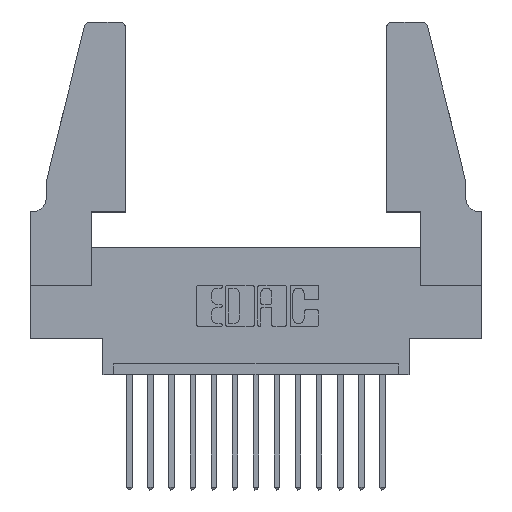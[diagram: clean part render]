
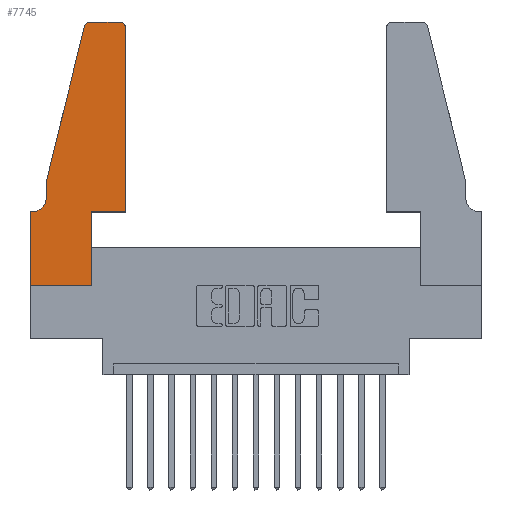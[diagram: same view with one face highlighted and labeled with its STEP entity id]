
A CAD part, top view. The second image highlights one B-rep face of the part: STEP entity #7745.
In plain terms, the highlighted planar face has unit normal (0, 0, 1).
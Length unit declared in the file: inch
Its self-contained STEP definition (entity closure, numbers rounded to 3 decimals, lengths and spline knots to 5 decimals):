
#63 = LINE ( 'NONE', #11155, #7960 ) ;
#189 = DIRECTION ( 'NONE',  ( 1., 0., 0. ) ) ;
#231 = ORIENTED_EDGE ( 'NONE', *, *, #7667, .T. ) ;
#413 = EDGE_CURVE ( 'NONE', #4228, #542, #7952, .T. ) ;
#529 = DIRECTION ( 'NONE',  ( -1., 0., 0. ) ) ;
#542 = VERTEX_POINT ( 'NONE', #15100 ) ;
#608 = EDGE_CURVE ( 'NONE', #13266, #11403, #9667, .T. ) ;
#725 = LINE ( 'NONE', #15301, #3039 ) ;
#782 = VECTOR ( 'NONE', #9727, 39.37008 ) ;
#928 = DIRECTION ( 'NONE',  ( 0., 0., 1. ) ) ;
#932 = AXIS2_PLACEMENT_3D ( 'NONE', #10779, #1033, #7289 ) ;
#1033 = DIRECTION ( 'NONE',  ( 0., 0., 1. ) ) ;
#1196 = DIRECTION ( 'NONE',  ( 0., -1., 0. ) ) ;
#1486 = VERTEX_POINT ( 'NONE', #13986 ) ;
#1506 = ORIENTED_EDGE ( 'NONE', *, *, #13818, .T. ) ;
#1510 = VECTOR ( 'NONE', #1196, 39.37008 ) ;
#1720 = DIRECTION ( 'NONE',  ( 0., 1., 0. ) ) ;
#1723 = VECTOR ( 'NONE', #12446, 39.37008 ) ;
#1784 = DIRECTION ( 'NONE',  ( 0., 0., -1. ) ) ;
#2279 = DIRECTION ( 'NONE',  ( 0., 1., 0. ) ) ;
#2294 = LINE ( 'NONE', #2817, #1723 ) ;
#2319 = CARTESIAN_POINT ( 'NONE',  ( 0.284, 1.22, 0.37 ) ) ;
#2699 = PLANE ( 'NONE',  #932 ) ;
#2817 = CARTESIAN_POINT ( 'NONE',  ( 0., 0., 0.37 ) ) ;
#2874 = LINE ( 'NONE', #2894, #12319 ) ;
#2894 = CARTESIAN_POINT ( 'NONE',  ( 0.4505, 0.35, 0.37 ) ) ;
#3039 = VECTOR ( 'NONE', #529, 39.37008 ) ;
#3141 = CARTESIAN_POINT ( 'NONE',  ( 0.2865, 0., 0.37 ) ) ;
#3272 = LINE ( 'NONE', #9671, #782 ) ;
#3279 = VERTEX_POINT ( 'NONE', #13109 ) ;
#3330 = CARTESIAN_POINT ( 'NONE',  ( 0.2865, 0.35, 0.37 ) ) ;
#3629 = CIRCLE ( 'NONE', #12653, 0.03 ) ;
#3825 = ORIENTED_EDGE ( 'NONE', *, *, #15422, .T. ) ;
#4015 = CARTESIAN_POINT ( 'NONE',  ( 0.0755, 0.5, 0.37 ) ) ;
#4043 = DIRECTION ( 'NONE',  ( -1., 0., 0. ) ) ;
#4045 = VERTEX_POINT ( 'NONE', #4311 ) ;
#4228 = VERTEX_POINT ( 'NONE', #7451 ) ;
#4311 = CARTESIAN_POINT ( 'NONE',  ( 0.4205, 1.25, 0.37 ) ) ;
#4902 = ORIENTED_EDGE ( 'NONE', *, *, #12905, .T. ) ;
#4983 = AXIS2_PLACEMENT_3D ( 'NONE', #2319, #928, #12179 ) ;
#5241 = EDGE_CURVE ( 'NONE', #542, #13461, #63, .T. ) ;
#5248 = CARTESIAN_POINT ( 'NONE',  ( 0.4205, 1.22, 0.37 ) ) ;
#5386 = LINE ( 'NONE', #8455, #1510 ) ;
#5908 = LINE ( 'NONE', #15460, #12884 ) ;
#6015 = DIRECTION ( 'NONE',  ( -0.239, -0.971, 0. ) ) ;
#6518 = FACE_OUTER_BOUND ( 'NONE', #14135, .T. ) ;
#7149 = CARTESIAN_POINT ( 'NONE',  ( 0.4505, 0.35, 0.37 ) ) ;
#7289 = DIRECTION ( 'NONE',  ( 1., 0., 0. ) ) ;
#7338 = ORIENTED_EDGE ( 'NONE', *, *, #13705, .T. ) ;
#7344 = ORIENTED_EDGE ( 'NONE', *, *, #12371, .T. ) ;
#7451 = CARTESIAN_POINT ( 'NONE',  ( 0.284, 1.25, 0.37 ) ) ;
#7667 = EDGE_CURVE ( 'NONE', #12874, #9202, #3272, .T. ) ;
#7682 = AXIS2_PLACEMENT_3D ( 'NONE', #9146, #1784, #15384 ) ;
#7745 = ADVANCED_FACE ( 'NONE', ( #6518 ), #2699, .T. ) ;
#7828 = DIRECTION ( 'NONE',  ( 1., 0., 0. ) ) ;
#7952 = CIRCLE ( 'NONE', #4983, 0.03 ) ;
#7960 = VECTOR ( 'NONE', #6015, 39.37008 ) ;
#8149 = VECTOR ( 'NONE', #1720, 39.37008 ) ;
#8455 = CARTESIAN_POINT ( 'NONE',  ( 0.0755, 0.5, 0.37 ) ) ;
#8996 = VERTEX_POINT ( 'NONE', #15156 ) ;
#9056 = ORIENTED_EDGE ( 'NONE', *, *, #12890, .T. ) ;
#9146 = CARTESIAN_POINT ( 'NONE',  ( 0.0055, 0.42, 0.37 ) ) ;
#9202 = VERTEX_POINT ( 'NONE', #11479 ) ;
#9304 = CARTESIAN_POINT ( 'NONE',  ( 0.4505, 1.22, 0.37 ) ) ;
#9667 = LINE ( 'NONE', #3330, #8149 ) ;
#9671 = CARTESIAN_POINT ( 'NONE',  ( 0., 0., 0.37 ) ) ;
#9727 = DIRECTION ( 'NONE',  ( 0., -1., 0. ) ) ;
#10391 = VECTOR ( 'NONE', #2279, 39.37008 ) ;
#10779 = CARTESIAN_POINT ( 'NONE',  ( 0., 0.35, 0.37 ) ) ;
#11059 = ORIENTED_EDGE ( 'NONE', *, *, #608, .T. ) ;
#11155 = CARTESIAN_POINT ( 'NONE',  ( 0.0755, 0.5, 0.37 ) ) ;
#11343 = CARTESIAN_POINT ( 'NONE',  ( 0., 0.35, 0.37 ) ) ;
#11390 = ORIENTED_EDGE ( 'NONE', *, *, #5241, .T. ) ;
#11403 = VERTEX_POINT ( 'NONE', #13115 ) ;
#11468 = VERTEX_POINT ( 'NONE', #9304 ) ;
#11479 = CARTESIAN_POINT ( 'NONE',  ( 0., 0., 0.37 ) ) ;
#11537 = ORIENTED_EDGE ( 'NONE', *, *, #12830, .T. ) ;
#12179 = DIRECTION ( 'NONE',  ( 1., 0., 0. ) ) ;
#12319 = VECTOR ( 'NONE', #7828, 39.37008 ) ;
#12371 = EDGE_CURVE ( 'NONE', #3279, #1486, #14083, .T. ) ;
#12422 = DIRECTION ( 'NONE',  ( 0., 0., 1. ) ) ;
#12446 = DIRECTION ( 'NONE',  ( 1., 0., 0. ) ) ;
#12506 = LINE ( 'NONE', #7149, #10391 ) ;
#12653 = AXIS2_PLACEMENT_3D ( 'NONE', #5248, #12422, #189 ) ;
#12830 = EDGE_CURVE ( 'NONE', #13461, #3279, #5386, .T. ) ;
#12874 = VERTEX_POINT ( 'NONE', #11343 ) ;
#12884 = VECTOR ( 'NONE', #4043, 39.37008 ) ;
#12890 = EDGE_CURVE ( 'NONE', #9202, #13266, #2294, .T. ) ;
#12905 = EDGE_CURVE ( 'NONE', #8996, #11468, #12506, .T. ) ;
#13109 = CARTESIAN_POINT ( 'NONE',  ( 0.0755, 0.42, 0.37 ) ) ;
#13115 = CARTESIAN_POINT ( 'NONE',  ( 0.2865, 0.35, 0.37 ) ) ;
#13266 = VERTEX_POINT ( 'NONE', #3141 ) ;
#13461 = VERTEX_POINT ( 'NONE', #4015 ) ;
#13609 = EDGE_CURVE ( 'NONE', #11468, #4045, #3629, .T. ) ;
#13705 = EDGE_CURVE ( 'NONE', #4045, #4228, #5908, .T. ) ;
#13818 = EDGE_CURVE ( 'NONE', #1486, #12874, #725, .T. ) ;
#13986 = CARTESIAN_POINT ( 'NONE',  ( 0.0055, 0.35, 0.37 ) ) ;
#14083 = CIRCLE ( 'NONE', #7682, 0.07 ) ;
#14135 = EDGE_LOOP ( 'NONE', ( #7338, #15339, #11390, #11537, #7344, #1506, #231, #9056, #11059, #3825, #4902, #14521 ) ) ;
#14521 = ORIENTED_EDGE ( 'NONE', *, *, #13609, .T. ) ;
#15100 = CARTESIAN_POINT ( 'NONE',  ( 0.25487, 1.22718, 0.37 ) ) ;
#15156 = CARTESIAN_POINT ( 'NONE',  ( 0.4505, 0.35, 0.37 ) ) ;
#15301 = CARTESIAN_POINT ( 'NONE',  ( 0.0755, 0.35, 0.37 ) ) ;
#15339 = ORIENTED_EDGE ( 'NONE', *, *, #413, .T. ) ;
#15384 = DIRECTION ( 'NONE',  ( -1., 0., 0. ) ) ;
#15422 = EDGE_CURVE ( 'NONE', #11403, #8996, #2874, .T. ) ;
#15460 = CARTESIAN_POINT ( 'NONE',  ( 0.2605, 1.25, 0.37 ) ) ;
